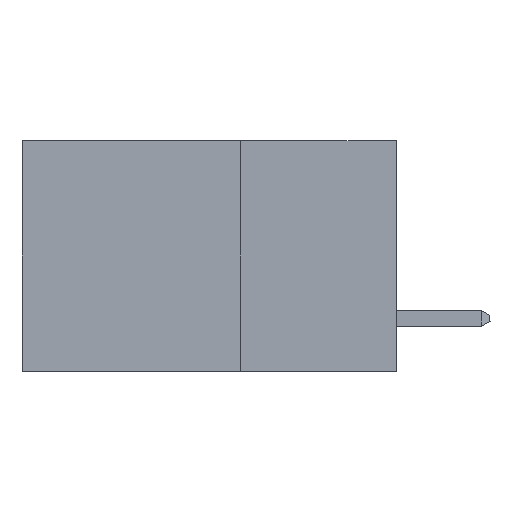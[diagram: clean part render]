
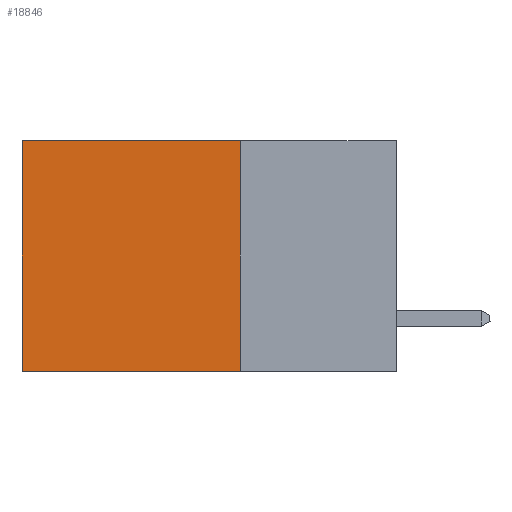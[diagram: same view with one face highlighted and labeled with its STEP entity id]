
A CAD part, left-side view. The second image highlights one B-rep face of the part: STEP entity #18846.
In plain terms, the highlighted planar face has unit normal (-1, 0, 0).
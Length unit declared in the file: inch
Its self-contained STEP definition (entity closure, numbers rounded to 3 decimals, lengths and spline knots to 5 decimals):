
#264 = CARTESIAN_POINT ( 'NONE',  ( 0.298, 0.6, 0. ) ) ;
#3170 = VERTEX_POINT ( 'NONE', #21014 ) ;
#3867 = LINE ( 'NONE', #264, #8750 ) ;
#3868 = VECTOR ( 'NONE', #15609, 39.37008 ) ;
#4649 = VERTEX_POINT ( 'NONE', #23505 ) ;
#4898 = AXIS2_PLACEMENT_3D ( 'NONE', #8855, #21645, #10764 ) ;
#4978 = CARTESIAN_POINT ( 'NONE',  ( 0.298, 0.25, 0. ) ) ;
#5591 = ORIENTED_EDGE ( 'NONE', *, *, #12215, .F. ) ;
#8232 = CARTESIAN_POINT ( 'NONE',  ( 0.298, 0.25, 0. ) ) ;
#8613 = EDGE_CURVE ( 'NONE', #16931, #10908, #11055, .T. ) ;
#8750 = VECTOR ( 'NONE', #20565, 39.37008 ) ;
#8855 = CARTESIAN_POINT ( 'NONE',  ( 0.298, 0.25, 0. ) ) ;
#10457 = VECTOR ( 'NONE', #12354, 39.37008 ) ;
#10764 = DIRECTION ( 'NONE',  ( 0., 0., -1. ) ) ;
#10908 = VERTEX_POINT ( 'NONE', #16065 ) ;
#11055 = LINE ( 'NONE', #4978, #10457 ) ;
#11144 = ORIENTED_EDGE ( 'NONE', *, *, #8613, .F. ) ;
#12215 = EDGE_CURVE ( 'NONE', #10908, #4649, #18970, .T. ) ;
#12354 = DIRECTION ( 'NONE',  ( 0., 0., -1. ) ) ;
#12548 = CARTESIAN_POINT ( 'NONE',  ( 0.298, 0.25, -0.37 ) ) ;
#14169 = VECTOR ( 'NONE', #18015, 39.37008 ) ;
#14208 = ORIENTED_EDGE ( 'NONE', *, *, #23039, .T. ) ;
#15609 = DIRECTION ( 'NONE',  ( 0., 1., 0. ) ) ;
#16065 = CARTESIAN_POINT ( 'NONE',  ( 0.298, 0.25, -0.37 ) ) ;
#16563 = EDGE_LOOP ( 'NONE', ( #14208, #5591, #11144, #18287 ) ) ;
#16931 = VERTEX_POINT ( 'NONE', #21388 ) ;
#18015 = DIRECTION ( 'NONE',  ( 0., 1., 0. ) ) ;
#18287 = ORIENTED_EDGE ( 'NONE', *, *, #20503, .T. ) ;
#18521 = LINE ( 'NONE', #8232, #3868 ) ;
#18846 = ADVANCED_FACE ( 'NONE', ( #23382 ), #19819, .F. ) ;
#18970 = LINE ( 'NONE', #12548, #14169 ) ;
#19819 = PLANE ( 'NONE',  #4898 ) ;
#20503 = EDGE_CURVE ( 'NONE', #16931, #3170, #18521, .T. ) ;
#20565 = DIRECTION ( 'NONE',  ( 0., 0., -1. ) ) ;
#21014 = CARTESIAN_POINT ( 'NONE',  ( 0.298, 0.6, 0. ) ) ;
#21388 = CARTESIAN_POINT ( 'NONE',  ( 0.298, 0.25, 0. ) ) ;
#21645 = DIRECTION ( 'NONE',  ( 1., 0., 0. ) ) ;
#23039 = EDGE_CURVE ( 'NONE', #3170, #4649, #3867, .T. ) ;
#23382 = FACE_OUTER_BOUND ( 'NONE', #16563, .T. ) ;
#23505 = CARTESIAN_POINT ( 'NONE',  ( 0.298, 0.6, -0.37 ) ) ;
